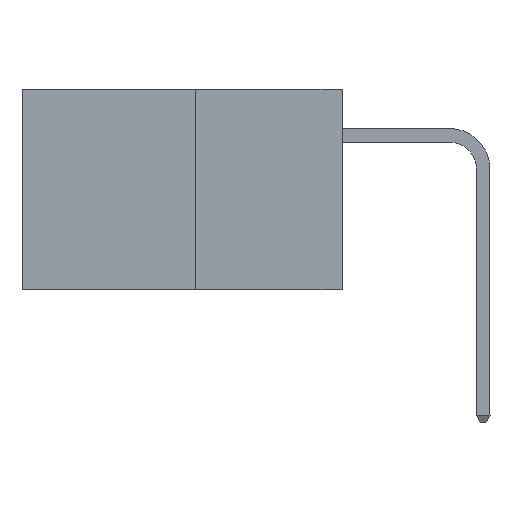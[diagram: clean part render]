
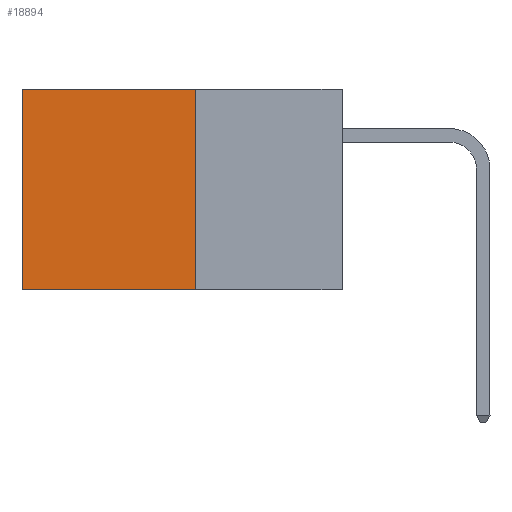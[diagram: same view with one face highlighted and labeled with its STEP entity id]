
A CAD part, left-side view. The second image highlights one B-rep face of the part: STEP entity #18894.
In plain terms, the highlighted planar face has unit normal (-1, 0, 0).
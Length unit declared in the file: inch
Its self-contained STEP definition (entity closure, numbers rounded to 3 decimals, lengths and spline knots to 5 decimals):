
#485 = DIRECTION ( 'NONE',  ( 0., 0., -1. ) ) ;
#1240 = ORIENTED_EDGE ( 'NONE', *, *, #3526, .F. ) ;
#1249 = DIRECTION ( 'NONE',  ( 0., 1., 0. ) ) ;
#1319 = LINE ( 'NONE', #5515, #24424 ) ;
#1459 = DIRECTION ( 'NONE',  ( 0., 1., 0. ) ) ;
#3526 = EDGE_CURVE ( 'NONE', #11220, #11925, #1319, .T. ) ;
#4887 = EDGE_CURVE ( 'NONE', #11925, #24605, #7269, .T. ) ;
#4949 = EDGE_CURVE ( 'NONE', #10831, #24605, #17025, .T. ) ;
#5515 = CARTESIAN_POINT ( 'NONE',  ( 0.277, 0.27, -0.37 ) ) ;
#6389 = PLANE ( 'NONE',  #7174 ) ;
#7174 = AXIS2_PLACEMENT_3D ( 'NONE', #21928, #8639, #24192 ) ;
#7269 = LINE ( 'NONE', #19329, #18411 ) ;
#7576 = ORIENTED_EDGE ( 'NONE', *, *, #4949, .T. ) ;
#8139 = VECTOR ( 'NONE', #1249, 39.37008 ) ;
#8639 = DIRECTION ( 'NONE',  ( 1., 0., 0. ) ) ;
#9106 = CARTESIAN_POINT ( 'NONE',  ( 0.277, 0.27, 0. ) ) ;
#9439 = CARTESIAN_POINT ( 'NONE',  ( 0.277, 0.59, 0. ) ) ;
#9776 = ORIENTED_EDGE ( 'NONE', *, *, #28889, .T. ) ;
#10129 = ORIENTED_EDGE ( 'NONE', *, *, #4887, .F. ) ;
#10831 = VERTEX_POINT ( 'NONE', #9439 ) ;
#11220 = VERTEX_POINT ( 'NONE', #9106 ) ;
#11925 = VERTEX_POINT ( 'NONE', #13743 ) ;
#12000 = CARTESIAN_POINT ( 'NONE',  ( 0.277, 0.59, -0.37 ) ) ;
#13743 = CARTESIAN_POINT ( 'NONE',  ( 0.277, 0.27, -0.37 ) ) ;
#14084 = DIRECTION ( 'NONE',  ( 0., 0., -1. ) ) ;
#14697 = CARTESIAN_POINT ( 'NONE',  ( 0.277, 0.27, 0. ) ) ;
#16760 = FACE_OUTER_BOUND ( 'NONE', #28646, .T. ) ;
#17025 = LINE ( 'NONE', #12000, #22209 ) ;
#18234 = CARTESIAN_POINT ( 'NONE',  ( 0.277, 0.59, -0.37 ) ) ;
#18411 = VECTOR ( 'NONE', #1459, 39.37008 ) ;
#18894 = ADVANCED_FACE ( 'NONE', ( #16760 ), #6389, .F. ) ;
#19329 = CARTESIAN_POINT ( 'NONE',  ( 0.277, 0.27, -0.37 ) ) ;
#20635 = LINE ( 'NONE', #14697, #8139 ) ;
#21928 = CARTESIAN_POINT ( 'NONE',  ( 0.277, 0.27, -0.37 ) ) ;
#22209 = VECTOR ( 'NONE', #485, 39.37008 ) ;
#24192 = DIRECTION ( 'NONE',  ( 0., 0., -1. ) ) ;
#24424 = VECTOR ( 'NONE', #14084, 39.37008 ) ;
#24605 = VERTEX_POINT ( 'NONE', #18234 ) ;
#28646 = EDGE_LOOP ( 'NONE', ( #7576, #10129, #1240, #9776 ) ) ;
#28889 = EDGE_CURVE ( 'NONE', #11220, #10831, #20635, .T. ) ;
